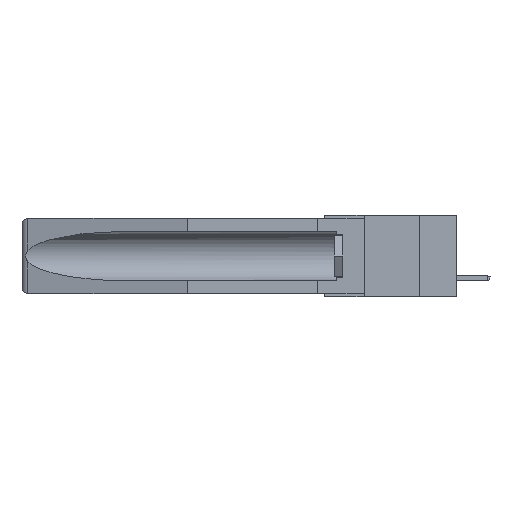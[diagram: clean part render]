
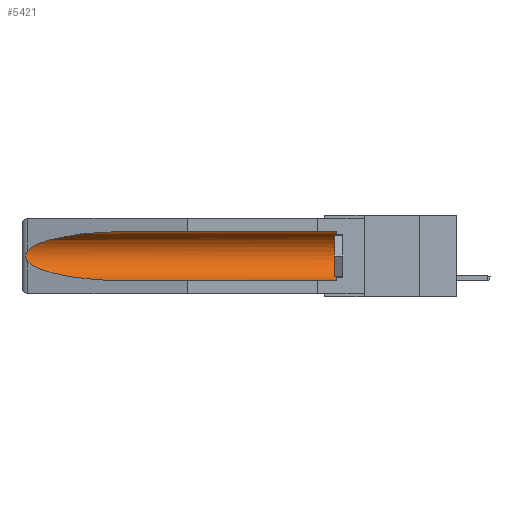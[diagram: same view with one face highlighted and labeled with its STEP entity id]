
A CAD part, left-side view. The second image highlights one B-rep face of the part: STEP entity #5421.
In plain terms, the highlighted cylindrical face has radius 2.857 mm (diameter 5.715 mm), a partial arc.
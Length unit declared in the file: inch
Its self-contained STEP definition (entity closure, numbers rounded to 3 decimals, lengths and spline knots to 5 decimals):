
#236 = DIRECTION ( 'NONE',  ( 0., 1., 0. ) ) ;
#341 = LINE ( 'NONE', #5070, #2980 ) ;
#665 = CARTESIAN_POINT ( 'NONE',  ( 0.25451, 1.48313, -0.09465 ) ) ;
#862 = CARTESIAN_POINT ( 'NONE',  ( 0.155, 0.126, -0.284 ) ) ;
#1672 = ORIENTED_EDGE ( 'NONE', *, *, #12032, .T. ) ;
#2443 = VERTEX_POINT ( 'NONE', #6815 ) ;
#2980 = VECTOR ( 'NONE', #17159, 39.37008 ) ;
#4028 = CARTESIAN_POINT ( 'NONE',  ( 0.26654, 1.53092, -0.15636 ) ) ;
#4512 = CARTESIAN_POINT ( 'NONE',  ( 0.26537, 1.52718, -0.19328 ) ) ;
#5070 = CARTESIAN_POINT ( 'NONE',  ( 0.155, -0.30754, -0.059 ) ) ;
#5421 = ADVANCED_FACE ( 'NONE', ( #21822 ), #22570, .F. ) ;
#5837 = AXIS2_PLACEMENT_3D ( 'NONE', #28749, #31073, #16086 ) ;
#6156 = EDGE_LOOP ( 'NONE', ( #1672, #19996, #25833, #24695, #8529, #23180 ) ) ;
#6815 = CARTESIAN_POINT ( 'NONE',  ( 0.155, 0.126, -0.059 ) ) ;
#8121 = CARTESIAN_POINT ( 'NONE',  ( 0.21114, 1.30732, -0.059 ) ) ;
#8529 = ORIENTED_EDGE ( 'NONE', *, *, #17340, .T. ) ;
#8659 = CARTESIAN_POINT ( 'NONE',  ( 0.155, 1.07973, -0.284 ) ) ;
#9487 =( BOUNDED_CURVE ( )  B_SPLINE_CURVE ( 3, ( #20378, #23034, #28037, #8659 ),
 .UNSPECIFIED., .F., .T. ) 
 B_SPLINE_CURVE_WITH_KNOTS ( ( 4, 4 ),
 ( 0.1948, 1.5708 ),
 .UNSPECIFIED. ) 
 CURVE ( )  GEOMETRIC_REPRESENTATION_ITEM ( )  RATIONAL_B_SPLINE_CURVE ( ( 1., 0.848, 0.848, 1. ) ) 
 REPRESENTATION_ITEM ( '' )  );
#9970 = DIRECTION ( 'NONE',  ( 0., 1., 0. ) ) ;
#10685 = VERTEX_POINT ( 'NONE', #15791 ) ;
#11191 = CARTESIAN_POINT ( 'NONE',  ( 0.26655, 1.53094, -0.18657 ) ) ;
#11283 = CARTESIAN_POINT ( 'NONE',  ( 0.26597, 1.5296, -0.19026 ) ) ;
#11473 = VERTEX_POINT ( 'NONE', #862 ) ;
#11701 = LINE ( 'NONE', #19552, #26882 ) ;
#12032 = EDGE_CURVE ( 'NONE', #29579, #28411, #12732, .T. ) ;
#12365 = CARTESIAN_POINT ( 'NONE',  ( 0.155, -0.30754, -0.1715 ) ) ;
#12732 =( BOUNDED_CURVE ( )  B_SPLINE_CURVE ( 3, ( #25131, #8121, #665, #20137 ),
 .UNSPECIFIED., .F., .F. ) 
 B_SPLINE_CURVE_WITH_KNOTS ( ( 4, 4 ),
 ( 4.71239, 6.08839 ),
 .UNSPECIFIED. ) 
 CURVE ( )  GEOMETRIC_REPRESENTATION_ITEM ( )  RATIONAL_B_SPLINE_CURVE ( ( 1., 0.848, 0.848, 1. ) ) 
 REPRESENTATION_ITEM ( '' )  );
#13056 = CIRCLE ( 'NONE', #5837, 0.1125 ) ;
#15296 = CARTESIAN_POINT ( 'NONE',  ( 0.26537, 1.52718, -0.14972 ) ) ;
#15791 = CARTESIAN_POINT ( 'NONE',  ( 0.155, 1.07973, -0.284 ) ) ;
#16086 = DIRECTION ( 'NONE',  ( 0., 0., 1. ) ) ;
#17159 = DIRECTION ( 'NONE',  ( 0., 1., 0. ) ) ;
#17340 = EDGE_CURVE ( 'NONE', #11473, #2443, #13056, .T. ) ;
#18247 = CARTESIAN_POINT ( 'NONE',  ( 0.2675, 1.53308, -0.17534 ) ) ;
#18458 = CARTESIAN_POINT ( 'NONE',  ( 0.2673, 1.53269, -0.17917 ) ) ;
#19552 = CARTESIAN_POINT ( 'NONE',  ( 0.155, -0.30754, -0.284 ) ) ;
#19786 = DIRECTION ( 'NONE',  ( 0., 0., 1. ) ) ;
#19996 = ORIENTED_EDGE ( 'NONE', *, *, #29017, .T. ) ;
#20137 = CARTESIAN_POINT ( 'NONE',  ( 0.26537, 1.52718, -0.14972 ) ) ;
#20378 = CARTESIAN_POINT ( 'NONE',  ( 0.26537, 1.52718, -0.19328 ) ) ;
#20839 = CARTESIAN_POINT ( 'NONE',  ( 0.26597, 1.52961, -0.15275 ) ) ;
#20952 = CARTESIAN_POINT ( 'NONE',  ( 0.26537, 1.52718, -0.19328 ) ) ;
#21315 = CARTESIAN_POINT ( 'NONE',  ( 0.155, 1.07973, -0.059 ) ) ;
#21822 = FACE_OUTER_BOUND ( 'NONE', #6156, .T. ) ;
#22570 = CYLINDRICAL_SURFACE ( 'NONE', #23029, 0.1125 ) ;
#23029 = AXIS2_PLACEMENT_3D ( 'NONE', #12365, #9970, #19786 ) ;
#23034 = CARTESIAN_POINT ( 'NONE',  ( 0.25451, 1.48313, -0.24835 ) ) ;
#23180 = ORIENTED_EDGE ( 'NONE', *, *, #25799, .T. ) ;
#24510 = EDGE_CURVE ( 'NONE', #11473, #10685, #11701, .T. ) ;
#24695 = ORIENTED_EDGE ( 'NONE', *, *, #24510, .F. ) ;
#25131 = CARTESIAN_POINT ( 'NONE',  ( 0.155, 1.07973, -0.059 ) ) ;
#25357 = EDGE_CURVE ( 'NONE', #27733, #10685, #9487, .T. ) ;
#25400 = CARTESIAN_POINT ( 'NONE',  ( 0.2673, 1.5327, -0.16383 ) ) ;
#25799 = EDGE_CURVE ( 'NONE', #2443, #29579, #341, .T. ) ;
#25833 = ORIENTED_EDGE ( 'NONE', *, *, #25357, .T. ) ;
#26882 = VECTOR ( 'NONE', #236, 39.37008 ) ;
#26956 = B_SPLINE_CURVE_WITH_KNOTS ( 'NONE', 3,
 ( #15296, #20839, #4028, #25400, #30379, #18247, #18458, #11191, #11283, #20952 ),
 .UNSPECIFIED., .F., .F.,
 ( 4, 2, 2, 2, 4 ),
 ( 0., 0.00029, 0.00058, 0.00087, 0.00117 ),
 .UNSPECIFIED. ) ;
#27733 = VERTEX_POINT ( 'NONE', #4512 ) ;
#28037 = CARTESIAN_POINT ( 'NONE',  ( 0.21114, 1.30732, -0.284 ) ) ;
#28411 = VERTEX_POINT ( 'NONE', #29710 ) ;
#28749 = CARTESIAN_POINT ( 'NONE',  ( 0.155, 0.126, -0.1715 ) ) ;
#29017 = EDGE_CURVE ( 'NONE', #28411, #27733, #26956, .T. ) ;
#29579 = VERTEX_POINT ( 'NONE', #21315 ) ;
#29710 = CARTESIAN_POINT ( 'NONE',  ( 0.26537, 1.52718, -0.14972 ) ) ;
#30379 = CARTESIAN_POINT ( 'NONE',  ( 0.2675, 1.53308, -0.16763 ) ) ;
#31073 = DIRECTION ( 'NONE',  ( 0., -1., 0. ) ) ;
